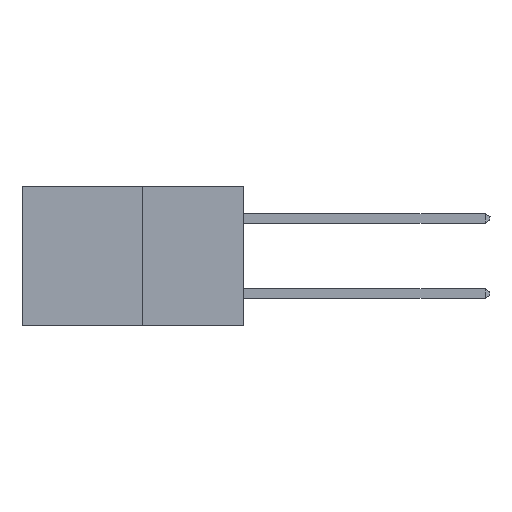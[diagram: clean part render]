
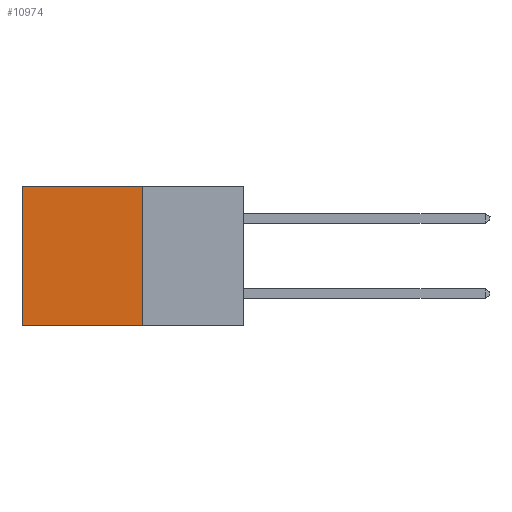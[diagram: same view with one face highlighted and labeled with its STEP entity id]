
A CAD part, left-side view. The second image highlights one B-rep face of the part: STEP entity #10974.
In plain terms, the highlighted planar face has unit normal (-1, 0, 0).
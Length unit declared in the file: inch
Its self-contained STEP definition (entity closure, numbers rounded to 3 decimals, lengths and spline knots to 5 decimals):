
#571 = CARTESIAN_POINT ( 'NONE',  ( 0.277, 0.59, 0. ) ) ;
#1467 = EDGE_CURVE ( 'NONE', #17338, #17073, #9255, .T. ) ;
#1533 = DIRECTION ( 'NONE',  ( 0., 0., -1. ) ) ;
#2071 = FACE_OUTER_BOUND ( 'NONE', #10962, .T. ) ;
#2072 = ORIENTED_EDGE ( 'NONE', *, *, #7885, .T. ) ;
#3140 = DIRECTION ( 'NONE',  ( 0., 0., -1. ) ) ;
#3229 = CARTESIAN_POINT ( 'NONE',  ( 0.277, 0.59, -0.37 ) ) ;
#3261 = ORIENTED_EDGE ( 'NONE', *, *, #12053, .F. ) ;
#3759 = PLANE ( 'NONE',  #15597 ) ;
#4113 = ORIENTED_EDGE ( 'NONE', *, *, #1467, .F. ) ;
#5169 = DIRECTION ( 'NONE',  ( 0., 1., 0. ) ) ;
#5625 = VECTOR ( 'NONE', #1533, 39.37008 ) ;
#5870 = LINE ( 'NONE', #6472, #9487 ) ;
#6108 = LINE ( 'NONE', #16041, #16498 ) ;
#6322 = VERTEX_POINT ( 'NONE', #571 ) ;
#6472 = CARTESIAN_POINT ( 'NONE',  ( 0.277, 0.27, -0.37 ) ) ;
#6557 = CARTESIAN_POINT ( 'NONE',  ( 0.277, 0.27, -0.37 ) ) ;
#6954 = ORIENTED_EDGE ( 'NONE', *, *, #15275, .T. ) ;
#7314 = LINE ( 'NONE', #14977, #14504 ) ;
#7874 = DIRECTION ( 'NONE',  ( 0., 1., 0. ) ) ;
#7885 = EDGE_CURVE ( 'NONE', #6322, #9118, #7314, .T. ) ;
#7948 = DIRECTION ( 'NONE',  ( 0., 0., -1. ) ) ;
#9053 = CARTESIAN_POINT ( 'NONE',  ( 0.277, 0.27, 0. ) ) ;
#9118 = VERTEX_POINT ( 'NONE', #3229 ) ;
#9255 = LINE ( 'NONE', #12631, #5625 ) ;
#9487 = VECTOR ( 'NONE', #7874, 39.37008 ) ;
#9941 = CARTESIAN_POINT ( 'NONE',  ( 0.277, 0.27, -0.37 ) ) ;
#10962 = EDGE_LOOP ( 'NONE', ( #2072, #3261, #4113, #6954 ) ) ;
#10974 = ADVANCED_FACE ( 'NONE', ( #2071 ), #3759, .F. ) ;
#12053 = EDGE_CURVE ( 'NONE', #17073, #9118, #5870, .T. ) ;
#12631 = CARTESIAN_POINT ( 'NONE',  ( 0.277, 0.27, -0.37 ) ) ;
#14504 = VECTOR ( 'NONE', #3140, 39.37008 ) ;
#14977 = CARTESIAN_POINT ( 'NONE',  ( 0.277, 0.59, -0.37 ) ) ;
#15275 = EDGE_CURVE ( 'NONE', #17338, #6322, #6108, .T. ) ;
#15597 = AXIS2_PLACEMENT_3D ( 'NONE', #6557, #16049, #7948 ) ;
#16041 = CARTESIAN_POINT ( 'NONE',  ( 0.277, 0.27, 0. ) ) ;
#16049 = DIRECTION ( 'NONE',  ( 1., 0., 0. ) ) ;
#16498 = VECTOR ( 'NONE', #5169, 39.37008 ) ;
#17073 = VERTEX_POINT ( 'NONE', #9941 ) ;
#17338 = VERTEX_POINT ( 'NONE', #9053 ) ;
